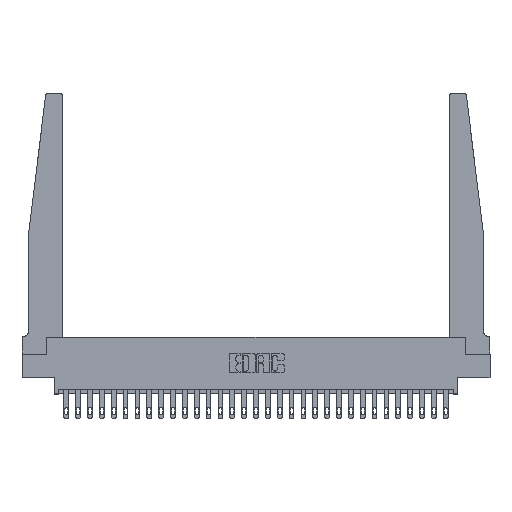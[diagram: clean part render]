
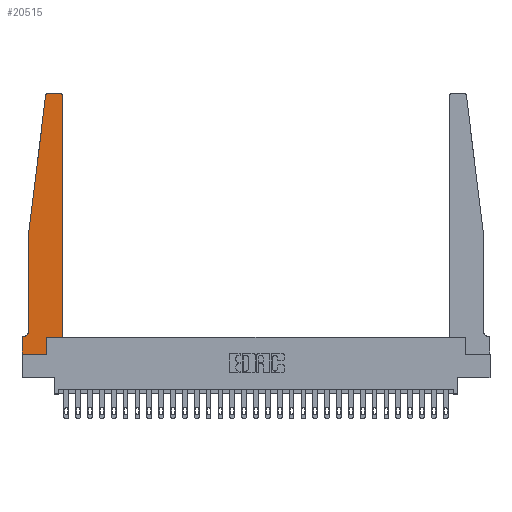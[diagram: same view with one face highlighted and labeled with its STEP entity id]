
A CAD part, top view. The second image highlights one B-rep face of the part: STEP entity #20515.
In plain terms, the highlighted planar face has unit normal (0, 0, 1).
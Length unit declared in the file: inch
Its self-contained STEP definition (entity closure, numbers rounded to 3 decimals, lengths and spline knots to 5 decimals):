
#263 = CARTESIAN_POINT ( 'NONE',  ( 0.25, 2.75, 0.37 ) ) ;
#272 = VERTEX_POINT ( 'NONE', #24772 ) ;
#891 = CARTESIAN_POINT ( 'NONE',  ( 0.425, 0.18, 0.37 ) ) ;
#1354 = DIRECTION ( 'NONE',  ( 1., 0., 0. ) ) ;
#2792 = VERTEX_POINT ( 'NONE', #7481 ) ;
#3191 = LINE ( 'NONE', #10105, #23746 ) ;
#3282 = VERTEX_POINT ( 'NONE', #24768 ) ;
#3463 = ORIENTED_EDGE ( 'NONE', *, *, #17353, .T. ) ;
#4003 = CARTESIAN_POINT ( 'NONE',  ( 0., 0.1875, 0.37 ) ) ;
#4011 = AXIS2_PLACEMENT_3D ( 'NONE', #26531, #8947, #17717 ) ;
#4057 = EDGE_CURVE ( 'NONE', #26441, #21810, #25225, .T. ) ;
#4333 = VERTEX_POINT ( 'NONE', #13549 ) ;
#5033 = EDGE_CURVE ( 'NONE', #5920, #4333, #3191, .T. ) ;
#5159 = CARTESIAN_POINT ( 'NONE',  ( 0., 0.1875, 0.37 ) ) ;
#5164 = CARTESIAN_POINT ( 'NONE',  ( 0.425, 0.18, 0.37 ) ) ;
#5353 = CARTESIAN_POINT ( 'NONE',  ( 0.065, 1.25, 0.37 ) ) ;
#5428 = DIRECTION ( 'NONE',  ( -0.122, -0.992, 0. ) ) ;
#5723 = EDGE_LOOP ( 'NONE', ( #23494, #12455, #20705, #17478, #22046, #3463, #24001, #22167, #19473, #27396, #27388, #24105 ) ) ;
#5920 = VERTEX_POINT ( 'NONE', #26665 ) ;
#6608 = CARTESIAN_POINT ( 'NONE',  ( 0.24675, 2.72367, 0.37 ) ) ;
#7361 = LINE ( 'NONE', #13879, #11020 ) ;
#7481 = CARTESIAN_POINT ( 'NONE',  ( 0.27653, 2.75, 0.37 ) ) ;
#7489 = CARTESIAN_POINT ( 'NONE',  ( 0.015, 0.1875, 0.37 ) ) ;
#7711 = CARTESIAN_POINT ( 'NONE',  ( 0.065, 0.1875, 0.37 ) ) ;
#7832 = DIRECTION ( 'NONE',  ( 0., 0., 1. ) ) ;
#8336 = VECTOR ( 'NONE', #8886, 39.37008 ) ;
#8886 = DIRECTION ( 'NONE',  ( -1., 0., 0. ) ) ;
#8947 = DIRECTION ( 'NONE',  ( 0., 0., -1. ) ) ;
#9592 = LINE ( 'NONE', #5353, #11618 ) ;
#9627 = CARTESIAN_POINT ( 'NONE',  ( 0.065, 1.25, 0.37 ) ) ;
#9844 = LINE ( 'NONE', #7711, #22381 ) ;
#9965 = CARTESIAN_POINT ( 'NONE',  ( 0.27653, 2.72, 0.37 ) ) ;
#10051 = EDGE_CURVE ( 'NONE', #2792, #11413, #16904, .T. ) ;
#10105 = CARTESIAN_POINT ( 'NONE',  ( 0., 0., 0.37 ) ) ;
#10130 = VECTOR ( 'NONE', #27512, 39.37008 ) ;
#10689 = EDGE_CURVE ( 'NONE', #4333, #12986, #12588, .T. ) ;
#11020 = VECTOR ( 'NONE', #24266, 39.37008 ) ;
#11413 = VERTEX_POINT ( 'NONE', #6608 ) ;
#11618 = VECTOR ( 'NONE', #17806, 39.37008 ) ;
#11962 = CARTESIAN_POINT ( 'NONE',  ( 0.2605, 0.18, 0.37 ) ) ;
#11984 = EDGE_CURVE ( 'NONE', #11413, #24125, #27412, .T. ) ;
#12445 = CARTESIAN_POINT ( 'NONE',  ( 0.2605, 0.18, 0.37 ) ) ;
#12455 = ORIENTED_EDGE ( 'NONE', *, *, #10051, .T. ) ;
#12588 = LINE ( 'NONE', #12445, #15001 ) ;
#12986 = VERTEX_POINT ( 'NONE', #11962 ) ;
#13141 = DIRECTION ( 'NONE',  ( 0., 0., 1. ) ) ;
#13549 = CARTESIAN_POINT ( 'NONE',  ( 0.2605, 0., 0.37 ) ) ;
#13641 = EDGE_CURVE ( 'NONE', #3282, #18954, #15323, .T. ) ;
#13879 = CARTESIAN_POINT ( 'NONE',  ( 0., 0., 0.37 ) ) ;
#14193 = CARTESIAN_POINT ( 'NONE',  ( 0.065, 1.25, 0.37 ) ) ;
#14519 = CARTESIAN_POINT ( 'NONE',  ( 0.425, 0.18, 0.37 ) ) ;
#14608 = FACE_OUTER_BOUND ( 'NONE', #5723, .T. ) ;
#14756 = EDGE_CURVE ( 'NONE', #19797, #5920, #7361, .T. ) ;
#14765 = AXIS2_PLACEMENT_3D ( 'NONE', #23908, #19359, #27899 ) ;
#15001 = VECTOR ( 'NONE', #18698, 39.37008 ) ;
#15079 = AXIS2_PLACEMENT_3D ( 'NONE', #9965, #7832, #26851 ) ;
#15323 = CIRCLE ( 'NONE', #4011, 0.05 ) ;
#15464 = EDGE_CURVE ( 'NONE', #272, #2792, #19670, .T. ) ;
#16904 = CIRCLE ( 'NONE', #15079, 0.03 ) ;
#17027 = CIRCLE ( 'NONE', #14765, 0.03 ) ;
#17353 = EDGE_CURVE ( 'NONE', #18954, #19797, #9844, .T. ) ;
#17399 = EDGE_CURVE ( 'NONE', #12986, #26441, #20750, .T. ) ;
#17478 = ORIENTED_EDGE ( 'NONE', *, *, #20713, .T. ) ;
#17717 = DIRECTION ( 'NONE',  ( -1., 0., 0. ) ) ;
#17806 = DIRECTION ( 'NONE',  ( 0., -1., 0. ) ) ;
#18698 = DIRECTION ( 'NONE',  ( 0., 1., 0. ) ) ;
#18954 = VERTEX_POINT ( 'NONE', #7489 ) ;
#19359 = DIRECTION ( 'NONE',  ( 0., 0., 1. ) ) ;
#19473 = ORIENTED_EDGE ( 'NONE', *, *, #10689, .T. ) ;
#19659 = EDGE_CURVE ( 'NONE', #21810, #272, #17027, .T. ) ;
#19670 = LINE ( 'NONE', #263, #8336 ) ;
#19797 = VERTEX_POINT ( 'NONE', #5159 ) ;
#20475 = DIRECTION ( 'NONE',  ( -1., 0., 0. ) ) ;
#20515 = ADVANCED_FACE ( 'NONE', ( #14608 ), #26340, .T. ) ;
#20705 = ORIENTED_EDGE ( 'NONE', *, *, #11984, .T. ) ;
#20713 = EDGE_CURVE ( 'NONE', #24125, #3282, #9592, .T. ) ;
#20750 = LINE ( 'NONE', #5164, #24200 ) ;
#21810 = VERTEX_POINT ( 'NONE', #25274 ) ;
#22046 = ORIENTED_EDGE ( 'NONE', *, *, #13641, .T. ) ;
#22167 = ORIENTED_EDGE ( 'NONE', *, *, #5033, .T. ) ;
#22381 = VECTOR ( 'NONE', #20475, 39.37008 ) ;
#22774 = VECTOR ( 'NONE', #5428, 39.37008 ) ;
#23428 = AXIS2_PLACEMENT_3D ( 'NONE', #4003, #13141, #27697 ) ;
#23494 = ORIENTED_EDGE ( 'NONE', *, *, #15464, .T. ) ;
#23746 = VECTOR ( 'NONE', #27434, 39.37008 ) ;
#23908 = CARTESIAN_POINT ( 'NONE',  ( 0.395, 2.72, 0.37 ) ) ;
#24001 = ORIENTED_EDGE ( 'NONE', *, *, #14756, .T. ) ;
#24105 = ORIENTED_EDGE ( 'NONE', *, *, #19659, .T. ) ;
#24125 = VERTEX_POINT ( 'NONE', #9627 ) ;
#24200 = VECTOR ( 'NONE', #1354, 39.37008 ) ;
#24266 = DIRECTION ( 'NONE',  ( 0., -1., 0. ) ) ;
#24768 = CARTESIAN_POINT ( 'NONE',  ( 0.065, 0.2375, 0.37 ) ) ;
#24772 = CARTESIAN_POINT ( 'NONE',  ( 0.395, 2.75, 0.37 ) ) ;
#25225 = LINE ( 'NONE', #891, #10130 ) ;
#25274 = CARTESIAN_POINT ( 'NONE',  ( 0.425, 2.72, 0.37 ) ) ;
#26340 = PLANE ( 'NONE',  #23428 ) ;
#26441 = VERTEX_POINT ( 'NONE', #14519 ) ;
#26531 = CARTESIAN_POINT ( 'NONE',  ( 0.015, 0.2375, 0.37 ) ) ;
#26665 = CARTESIAN_POINT ( 'NONE',  ( 0., 0., 0.37 ) ) ;
#26851 = DIRECTION ( 'NONE',  ( 1., 0., 0. ) ) ;
#27388 = ORIENTED_EDGE ( 'NONE', *, *, #4057, .T. ) ;
#27396 = ORIENTED_EDGE ( 'NONE', *, *, #17399, .T. ) ;
#27412 = LINE ( 'NONE', #14193, #22774 ) ;
#27434 = DIRECTION ( 'NONE',  ( 1., 0., 0. ) ) ;
#27512 = DIRECTION ( 'NONE',  ( 0., 1., 0. ) ) ;
#27697 = DIRECTION ( 'NONE',  ( 1., 0., 0. ) ) ;
#27899 = DIRECTION ( 'NONE',  ( 1., 0., 0. ) ) ;
